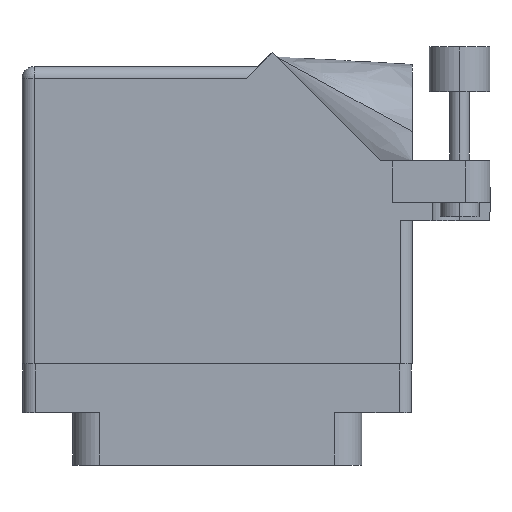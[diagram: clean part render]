
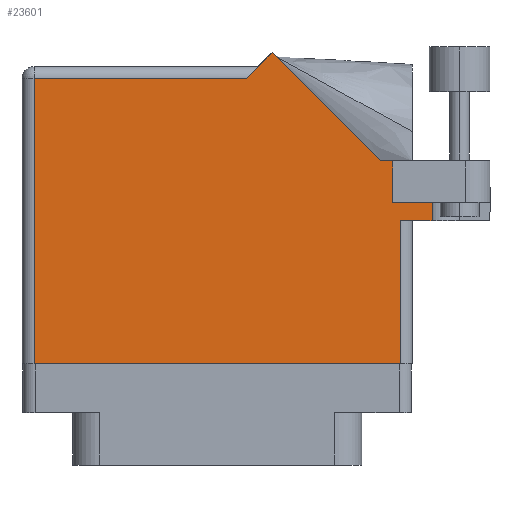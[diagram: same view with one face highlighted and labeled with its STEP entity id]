
A CAD part, front view. The second image highlights one B-rep face of the part: STEP entity #23601.
In plain terms, the highlighted face is planar.
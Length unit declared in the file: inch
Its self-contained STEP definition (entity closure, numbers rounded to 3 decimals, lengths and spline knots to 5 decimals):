
#326 = ORIENTED_EDGE ( 'NONE', *, *, #6328, .T. ) ;
#482 = DIRECTION ( 'NONE',  ( 0., -1., 0. ) ) ;
#636 = CARTESIAN_POINT ( 'NONE',  ( 0.15, 1.368, 0.455 ) ) ;
#923 = VERTEX_POINT ( 'NONE', #27021 ) ;
#928 = VECTOR ( 'NONE', #482, 39.37008 ) ;
#931 = VECTOR ( 'NONE', #31724, 39.37008 ) ;
#1103 = ORIENTED_EDGE ( 'NONE', *, *, #22322, .T. ) ;
#1576 = PLANE ( 'NONE',  #10515 ) ;
#1853 = DIRECTION ( 'NONE',  ( 1., 0., 0. ) ) ;
#2262 = LINE ( 'NONE', #11437, #928 ) ;
#3196 = VERTEX_POINT ( 'NONE', #9454 ) ;
#3224 = LINE ( 'NONE', #25495, #24708 ) ;
#3976 = DIRECTION ( 'NONE',  ( 0., -1., 0. ) ) ;
#4697 = LINE ( 'NONE', #34376, #20944 ) ;
#4965 = CARTESIAN_POINT ( 'NONE',  ( 1.1065, 0.637, 0.455 ) ) ;
#5297 = FACE_OUTER_BOUND ( 'NONE', #28819, .T. ) ;
#5311 = CARTESIAN_POINT ( 'NONE',  ( 0.943, -0.1, 0.455 ) ) ;
#5493 = ORIENTED_EDGE ( 'NONE', *, *, #16749, .T. ) ;
#5618 = EDGE_CURVE ( 'NONE', #27247, #11337, #5987, .T. ) ;
#5929 = VECTOR ( 'NONE', #13528, 39.37008 ) ;
#5987 = LINE ( 'NONE', #21348, #31926 ) ;
#6328 = EDGE_CURVE ( 'NONE', #3196, #30124, #34932, .T. ) ;
#6363 = EDGE_CURVE ( 'NONE', #6493, #923, #26120, .T. ) ;
#6493 = VERTEX_POINT ( 'NONE', #22626 ) ;
#7611 = LINE ( 'NONE', #17886, #21287 ) ;
#7635 = LINE ( 'NONE', #28822, #14671 ) ;
#7987 = CARTESIAN_POINT ( 'NONE',  ( 0.905, 0.731, 0.455 ) ) ;
#8548 = EDGE_CURVE ( 'NONE', #23528, #27247, #19901, .T. ) ;
#9454 = CARTESIAN_POINT ( 'NONE',  ( 0.905, 0.944, 0.455 ) ) ;
#10515 = AXIS2_PLACEMENT_3D ( 'NONE', #20949, #26568, #21072 ) ;
#10891 = ORIENTED_EDGE ( 'NONE', *, *, #31045, .T. ) ;
#10931 = DIRECTION ( 'NONE',  ( -1., 0., 0. ) ) ;
#11016 = LINE ( 'NONE', #13872, #16349 ) ;
#11337 = VERTEX_POINT ( 'NONE', #5311 ) ;
#11437 = CARTESIAN_POINT ( 'NONE',  ( 1.1065, 1.06177, 0.455 ) ) ;
#12048 = CARTESIAN_POINT ( 'NONE',  ( 0.83942, 0.944, 0.455 ) ) ;
#13528 = DIRECTION ( 'NONE',  ( 1., 0., 0. ) ) ;
#13872 = CARTESIAN_POINT ( 'NONE',  ( 0.212, 1.43, 0.455 ) ) ;
#14649 = ORIENTED_EDGE ( 'NONE', *, *, #23568, .F. ) ;
#14671 = VECTOR ( 'NONE', #17338, 39.37008 ) ;
#14773 = DIRECTION ( 'NONE',  ( 0., 1., 0. ) ) ;
#15467 = ORIENTED_EDGE ( 'NONE', *, *, #8548, .T. ) ;
#16182 = CARTESIAN_POINT ( 'NONE',  ( 1.405, 0.944, 0.455 ) ) ;
#16349 = VECTOR ( 'NONE', #28356, 39.37008 ) ;
#16749 = EDGE_CURVE ( 'NONE', #6493, #3196, #7611, .T. ) ;
#16950 = VERTEX_POINT ( 'NONE', #32942 ) ;
#17338 = DIRECTION ( 'NONE',  ( 1., 0., 0. ) ) ;
#17886 = CARTESIAN_POINT ( 'NONE',  ( 0.905, 0.731, 0.455 ) ) ;
#19072 = EDGE_CURVE ( 'NONE', #30124, #23550, #23296, .T. ) ;
#19171 = ORIENTED_EDGE ( 'NONE', *, *, #35783, .T. ) ;
#19542 = VECTOR ( 'NONE', #10931, 39.37008 ) ;
#19901 = LINE ( 'NONE', #21023, #31748 ) ;
#20944 = VECTOR ( 'NONE', #31444, 39.37008 ) ;
#20949 = CARTESIAN_POINT ( 'NONE',  ( -1.005, 1.43, 0.455 ) ) ;
#21023 = CARTESIAN_POINT ( 'NONE',  ( -0.943, -0.1, 0.455 ) ) ;
#21072 = DIRECTION ( 'NONE',  ( -1., 0., 0. ) ) ;
#21287 = VECTOR ( 'NONE', #14773, 39.37008 ) ;
#21335 = CARTESIAN_POINT ( 'NONE',  ( 0.83942, 0.944, 0.455 ) ) ;
#21348 = CARTESIAN_POINT ( 'NONE',  ( -1.005, -0.1, 0.455 ) ) ;
#21638 = ORIENTED_EDGE ( 'NONE', *, *, #19072, .T. ) ;
#22322 = EDGE_CURVE ( 'NONE', #11337, #16950, #3224, .T. ) ;
#22626 = CARTESIAN_POINT ( 'NONE',  ( 0.905, 0.731, 0.455 ) ) ;
#22731 = ORIENTED_EDGE ( 'NONE', *, *, #5618, .T. ) ;
#23296 = LINE ( 'NONE', #12048, #931 ) ;
#23528 = VERTEX_POINT ( 'NONE', #31237 ) ;
#23550 = VERTEX_POINT ( 'NONE', #33694 ) ;
#23568 = EDGE_CURVE ( 'NONE', #923, #32795, #2262, .T. ) ;
#23601 = ADVANCED_FACE ( 'NONE', ( #5297 ), #1576, .F. ) ;
#24708 = VECTOR ( 'NONE', #25614, 39.37008 ) ;
#25495 = CARTESIAN_POINT ( 'NONE',  ( 0.943, 0.637, 0.455 ) ) ;
#25614 = DIRECTION ( 'NONE',  ( 0., 1., 0. ) ) ;
#26120 = LINE ( 'NONE', #7987, #5929 ) ;
#26568 = DIRECTION ( 'NONE',  ( 0., 0., -1. ) ) ;
#27021 = CARTESIAN_POINT ( 'NONE',  ( 1.1065, 0.731, 0.455 ) ) ;
#27247 = VERTEX_POINT ( 'NONE', #34505 ) ;
#28356 = DIRECTION ( 'NONE',  ( -0.707, -0.707, 0. ) ) ;
#28819 = EDGE_LOOP ( 'NONE', ( #22731, #1103, #29808, #14649, #29726, #5493, #326, #21638, #19171, #10891, #15467 ) ) ;
#28822 = CARTESIAN_POINT ( 'NONE',  ( 1.005, 0.637, 0.455 ) ) ;
#28860 = VERTEX_POINT ( 'NONE', #636 ) ;
#29726 = ORIENTED_EDGE ( 'NONE', *, *, #6363, .F. ) ;
#29808 = ORIENTED_EDGE ( 'NONE', *, *, #31900, .T. ) ;
#30124 = VERTEX_POINT ( 'NONE', #21335 ) ;
#31045 = EDGE_CURVE ( 'NONE', #28860, #23528, #4697, .T. ) ;
#31237 = CARTESIAN_POINT ( 'NONE',  ( -0.943, 1.368, 0.455 ) ) ;
#31444 = DIRECTION ( 'NONE',  ( -1., 0., 0. ) ) ;
#31724 = DIRECTION ( 'NONE',  ( -0.707, 0.707, 0. ) ) ;
#31748 = VECTOR ( 'NONE', #3976, 39.37008 ) ;
#31900 = EDGE_CURVE ( 'NONE', #16950, #32795, #7635, .T. ) ;
#31926 = VECTOR ( 'NONE', #1853, 39.37008 ) ;
#32795 = VERTEX_POINT ( 'NONE', #4965 ) ;
#32942 = CARTESIAN_POINT ( 'NONE',  ( 0.943, 0.637, 0.455 ) ) ;
#33694 = CARTESIAN_POINT ( 'NONE',  ( 0.28271, 1.50071, 0.455 ) ) ;
#34376 = CARTESIAN_POINT ( 'NONE',  ( -1.005, 1.368, 0.455 ) ) ;
#34505 = CARTESIAN_POINT ( 'NONE',  ( -0.943, -0.1, 0.455 ) ) ;
#34932 = LINE ( 'NONE', #16182, #19542 ) ;
#35783 = EDGE_CURVE ( 'NONE', #23550, #28860, #11016, .T. ) ;
